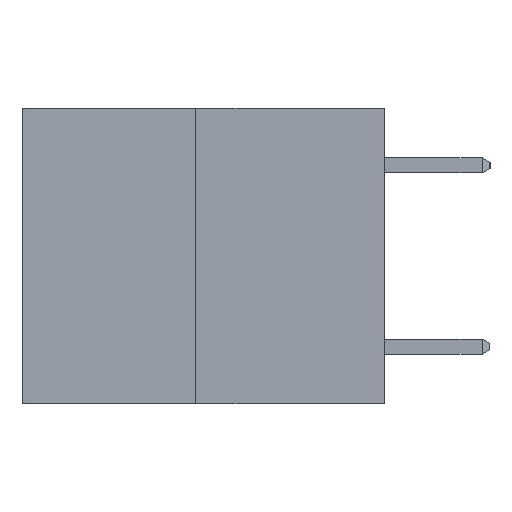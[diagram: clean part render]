
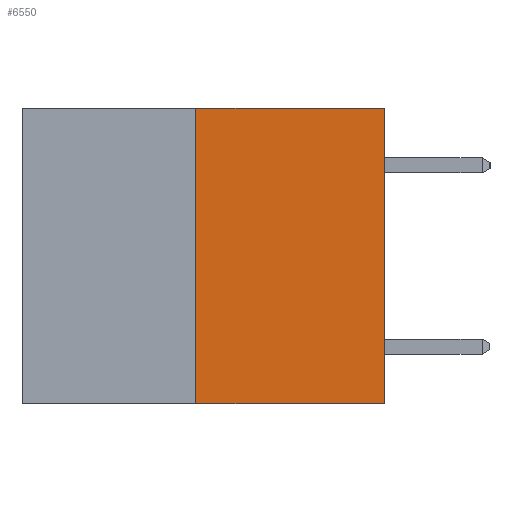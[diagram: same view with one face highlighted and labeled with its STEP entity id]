
A CAD part, left-side view. The second image highlights one B-rep face of the part: STEP entity #6550.
In plain terms, the highlighted planar face has unit normal (-1, 0, 0).
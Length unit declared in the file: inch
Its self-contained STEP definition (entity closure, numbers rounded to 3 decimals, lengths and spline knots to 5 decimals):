
#1279 = CARTESIAN_POINT ( 'NONE',  ( 0., 0.6, -0.49 ) ) ;
#1613 = ORIENTED_EDGE ( 'NONE', *, *, #6508, .F. ) ;
#1669 = LINE ( 'NONE', #1279, #5453 ) ;
#1811 = DIRECTION ( 'NONE',  ( 1., 0., 0. ) ) ;
#2295 = VECTOR ( 'NONE', #2478, 39.37008 ) ;
#2382 = VERTEX_POINT ( 'NONE', #3003 ) ;
#2411 = CARTESIAN_POINT ( 'NONE',  ( 0., 0.6, 0. ) ) ;
#2413 = FACE_OUTER_BOUND ( 'NONE', #4197, .T. ) ;
#2478 = DIRECTION ( 'NONE',  ( 0., -1., 0. ) ) ;
#2923 = DIRECTION ( 'NONE',  ( 0., 0., 1. ) ) ;
#3003 = CARTESIAN_POINT ( 'NONE',  ( 0., 0., -0.49 ) ) ;
#3066 = CARTESIAN_POINT ( 'NONE',  ( 0., 0.312, -0.49 ) ) ;
#3868 = DIRECTION ( 'NONE',  ( 0., 0., 1. ) ) ;
#4197 = EDGE_LOOP ( 'NONE', ( #8070, #5380, #5047, #1613 ) ) ;
#4241 = CARTESIAN_POINT ( 'NONE',  ( 0., 0.312, 0. ) ) ;
#4771 = VECTOR ( 'NONE', #2923, 39.37008 ) ;
#5047 = ORIENTED_EDGE ( 'NONE', *, *, #9640, .T. ) ;
#5252 = LINE ( 'NONE', #9617, #4771 ) ;
#5380 = ORIENTED_EDGE ( 'NONE', *, *, #8367, .T. ) ;
#5453 = VECTOR ( 'NONE', #9564, 39.37008 ) ;
#5547 = DIRECTION ( 'NONE',  ( 0., 0., -1. ) ) ;
#5611 = VERTEX_POINT ( 'NONE', #8927 ) ;
#6058 = CARTESIAN_POINT ( 'NONE',  ( 0., 0.312, -0.49 ) ) ;
#6357 = PLANE ( 'NONE',  #8291 ) ;
#6490 = VECTOR ( 'NONE', #3868, 39.37008 ) ;
#6508 = EDGE_CURVE ( 'NONE', #7801, #5611, #6893, .T. ) ;
#6550 = ADVANCED_FACE ( 'NONE', ( #2413 ), #6357, .F. ) ;
#6893 = LINE ( 'NONE', #2411, #2295 ) ;
#7466 = VERTEX_POINT ( 'NONE', #3066 ) ;
#7801 = VERTEX_POINT ( 'NONE', #4241 ) ;
#8070 = ORIENTED_EDGE ( 'NONE', *, *, #8640, .F. ) ;
#8291 = AXIS2_PLACEMENT_3D ( 'NONE', #8567, #1811, #5547 ) ;
#8367 = EDGE_CURVE ( 'NONE', #7466, #2382, #1669, .T. ) ;
#8483 = LINE ( 'NONE', #6058, #6490 ) ;
#8567 = CARTESIAN_POINT ( 'NONE',  ( 0., 0.6, 0. ) ) ;
#8640 = EDGE_CURVE ( 'NONE', #7466, #7801, #8483, .T. ) ;
#8927 = CARTESIAN_POINT ( 'NONE',  ( 0., 0., 0. ) ) ;
#9564 = DIRECTION ( 'NONE',  ( 0., -1., 0. ) ) ;
#9617 = CARTESIAN_POINT ( 'NONE',  ( 0., 0., 0. ) ) ;
#9640 = EDGE_CURVE ( 'NONE', #2382, #5611, #5252, .T. ) ;
